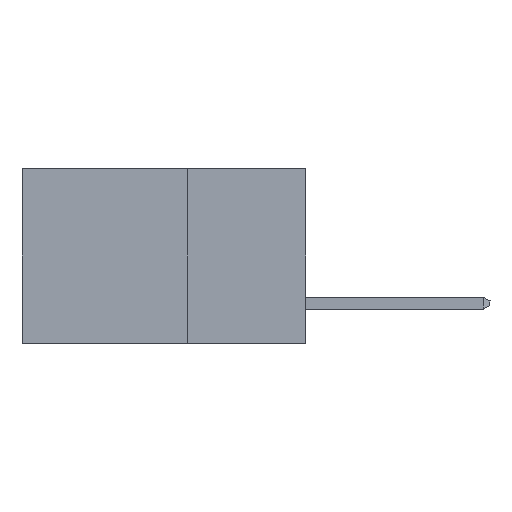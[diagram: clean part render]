
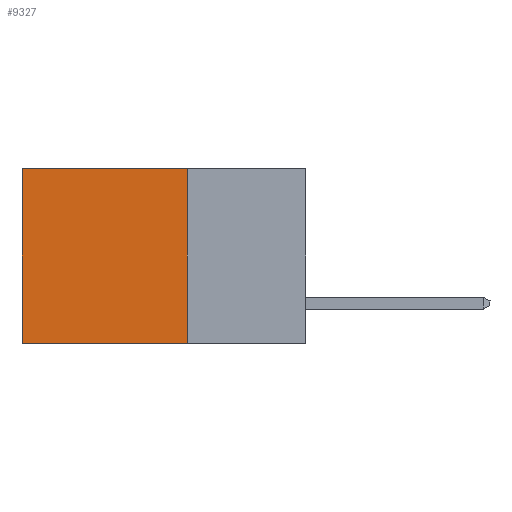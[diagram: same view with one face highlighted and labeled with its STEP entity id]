
A CAD part, left-side view. The second image highlights one B-rep face of the part: STEP entity #9327.
In plain terms, the highlighted planar face has unit normal (-1, 0, 0).
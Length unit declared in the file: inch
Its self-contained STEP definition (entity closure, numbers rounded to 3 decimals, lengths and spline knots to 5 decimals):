
#345 = CARTESIAN_POINT ( 'NONE',  ( 0.298, 0.25, 0. ) ) ;
#537 = DIRECTION ( 'NONE',  ( 0., 1., 0. ) ) ;
#571 = VECTOR ( 'NONE', #7362, 39.37008 ) ;
#789 = DIRECTION ( 'NONE',  ( 0., 1., 0. ) ) ;
#1668 = DIRECTION ( 'NONE',  ( 0., 0., -1. ) ) ;
#2407 = EDGE_CURVE ( 'NONE', #2467, #8279, #3641, .T. ) ;
#2467 = VERTEX_POINT ( 'NONE', #7933 ) ;
#2690 = CARTESIAN_POINT ( 'NONE',  ( 0.298, 0.6, 0. ) ) ;
#3641 = LINE ( 'NONE', #11891, #12007 ) ;
#3913 = LINE ( 'NONE', #14330, #571 ) ;
#4661 = EDGE_LOOP ( 'NONE', ( #7452, #5826, #11287, #4762 ) ) ;
#4762 = ORIENTED_EDGE ( 'NONE', *, *, #2407, .T. ) ;
#4771 = VECTOR ( 'NONE', #14112, 39.37008 ) ;
#4779 = LINE ( 'NONE', #13615, #6788 ) ;
#5116 = EDGE_CURVE ( 'NONE', #14908, #16101, #4779, .T. ) ;
#5347 = CARTESIAN_POINT ( 'NONE',  ( 0.298, 0.6, -0.37 ) ) ;
#5826 = ORIENTED_EDGE ( 'NONE', *, *, #5116, .F. ) ;
#6731 = PLANE ( 'NONE',  #7092 ) ;
#6788 = VECTOR ( 'NONE', #789, 39.37008 ) ;
#7092 = AXIS2_PLACEMENT_3D ( 'NONE', #345, #13019, #1668 ) ;
#7362 = DIRECTION ( 'NONE',  ( 0., 0., -1. ) ) ;
#7452 = ORIENTED_EDGE ( 'NONE', *, *, #9098, .T. ) ;
#7933 = CARTESIAN_POINT ( 'NONE',  ( 0.298, 0.25, 0. ) ) ;
#8279 = VERTEX_POINT ( 'NONE', #15144 ) ;
#9098 = EDGE_CURVE ( 'NONE', #8279, #16101, #14918, .T. ) ;
#9327 = ADVANCED_FACE ( 'NONE', ( #9526 ), #6731, .F. ) ;
#9526 = FACE_OUTER_BOUND ( 'NONE', #4661, .T. ) ;
#11287 = ORIENTED_EDGE ( 'NONE', *, *, #15509, .F. ) ;
#11891 = CARTESIAN_POINT ( 'NONE',  ( 0.298, 0.25, 0. ) ) ;
#12007 = VECTOR ( 'NONE', #537, 39.37008 ) ;
#13019 = DIRECTION ( 'NONE',  ( 1., 0., 0. ) ) ;
#13615 = CARTESIAN_POINT ( 'NONE',  ( 0.298, 0.25, -0.37 ) ) ;
#14112 = DIRECTION ( 'NONE',  ( 0., 0., -1. ) ) ;
#14330 = CARTESIAN_POINT ( 'NONE',  ( 0.298, 0.25, 0. ) ) ;
#14374 = CARTESIAN_POINT ( 'NONE',  ( 0.298, 0.25, -0.37 ) ) ;
#14908 = VERTEX_POINT ( 'NONE', #14374 ) ;
#14918 = LINE ( 'NONE', #2690, #4771 ) ;
#15144 = CARTESIAN_POINT ( 'NONE',  ( 0.298, 0.6, 0. ) ) ;
#15509 = EDGE_CURVE ( 'NONE', #2467, #14908, #3913, .T. ) ;
#16101 = VERTEX_POINT ( 'NONE', #5347 ) ;
